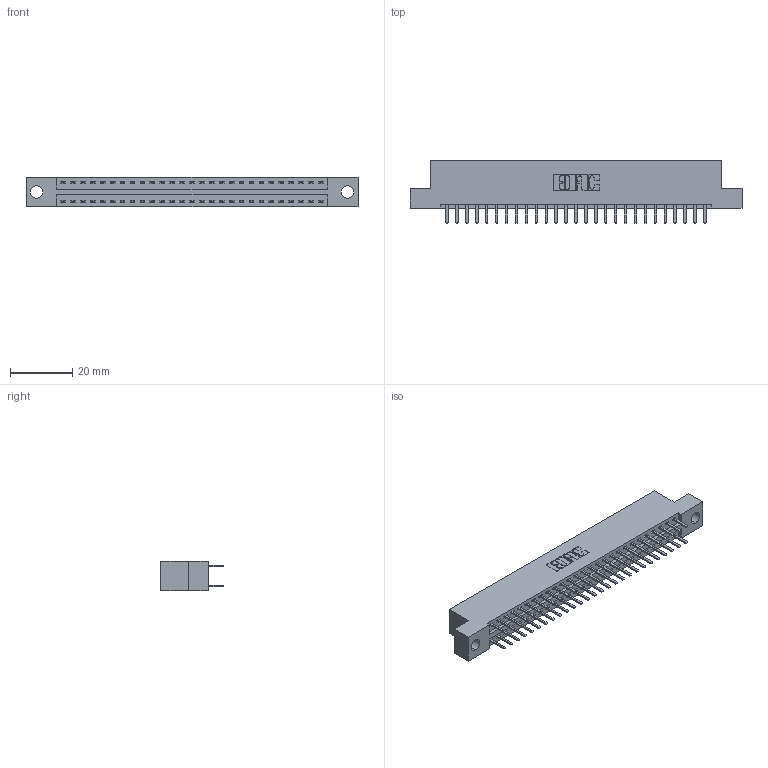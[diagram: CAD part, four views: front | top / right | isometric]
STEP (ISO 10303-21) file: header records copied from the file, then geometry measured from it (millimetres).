
FILE_DESCRIPTION (( 'STEP AP203' ), '1' );
FILE_NAME ('346-054-520-204.STEP', '2018-08-28T00:49:26', ( '' ), ( '' ), 'SwSTEP 2.0', 'SolidWorks 2016', '' );
FILE_SCHEMA (( 'CONFIG_CONTROL_DESIGN' ));
Length unit declared in the file: inch
Products named in the file (3): 346 Part_Flush Mounting Lugs - 0.156 Dia-TH; 345-292-001_345-293-120; 346-054-520-204
Assembly tree (55 placements, depth 2):
  346-054-520-204
    346 Part_Flush Mounting Lugs - 0.156 Dia-TH
    345-292-001_345-293-120  x54
Bounding box: 106.3 x 20.02 x 9.4 mm (x, y, z)
Volume: 10137.4 mm3; surface area: 13456.5 mm2
Topology: 55 solids, 55 shells, 3146 faces, 9131 edges, 5942 vertices
Faces by surface type: plane 2074, cylinder 1072
Entity records: 19757 total; most frequent: CARTESIAN_POINT 3288, ORIENTED_EDGE 3210, DIRECTION 2937, EDGE_CURVE 1605, LINE 1361, VECTOR 1361, VERTEX_POINT 1066, AXIS2_PLACEMENT_3D 788
